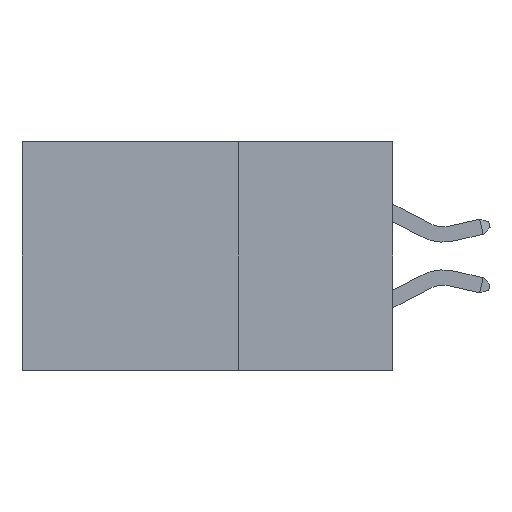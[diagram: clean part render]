
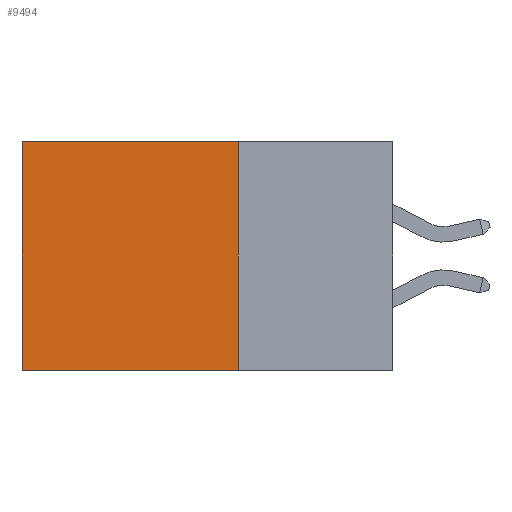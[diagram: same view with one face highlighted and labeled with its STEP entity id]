
A CAD part, left-side view. The second image highlights one B-rep face of the part: STEP entity #9494.
In plain terms, the highlighted planar face has unit normal (-1, 0, 0).
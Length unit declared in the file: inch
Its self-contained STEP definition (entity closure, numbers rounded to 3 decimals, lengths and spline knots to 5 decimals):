
#13 = CARTESIAN_POINT ( 'NONE',  ( 0.2875, 0.25, 0. ) ) ;
#37 = DIRECTION ( 'NONE',  ( 0., 0., -1. ) ) ;
#105 = ORIENTED_EDGE ( 'NONE', *, *, #1785, .T. ) ;
#1599 = EDGE_CURVE ( 'NONE', #8302, #7192, #10492, .T. ) ;
#1776 = VERTEX_POINT ( 'NONE', #13 ) ;
#1785 = EDGE_CURVE ( 'NONE', #1776, #11393, #3729, .T. ) ;
#2001 = LINE ( 'NONE', #6952, #3976 ) ;
#2182 = CARTESIAN_POINT ( 'NONE',  ( 0.2875, 0.25, -0.37 ) ) ;
#2454 = ORIENTED_EDGE ( 'NONE', *, *, #1599, .F. ) ;
#3083 = DIRECTION ( 'NONE',  ( 0., 1., 0. ) ) ;
#3729 = LINE ( 'NONE', #11576, #9092 ) ;
#3802 = DIRECTION ( 'NONE',  ( 0., 0., -1. ) ) ;
#3976 = VECTOR ( 'NONE', #7928, 39.37008 ) ;
#4517 = EDGE_CURVE ( 'NONE', #11393, #7192, #9019, .T. ) ;
#4982 = CARTESIAN_POINT ( 'NONE',  ( 0.2875, 0.25, -0.37 ) ) ;
#5694 = CARTESIAN_POINT ( 'NONE',  ( 0.2875, 0.25, 0. ) ) ;
#5913 = CARTESIAN_POINT ( 'NONE',  ( 0.2875, 0.6, 0. ) ) ;
#6952 = CARTESIAN_POINT ( 'NONE',  ( 0.2875, 0.25, 0. ) ) ;
#7192 = VERTEX_POINT ( 'NONE', #9740 ) ;
#7623 = PLANE ( 'NONE',  #8102 ) ;
#7928 = DIRECTION ( 'NONE',  ( 0., 0., -1. ) ) ;
#8092 = VECTOR ( 'NONE', #3083, 39.37008 ) ;
#8102 = AXIS2_PLACEMENT_3D ( 'NONE', #5694, #9473, #3802 ) ;
#8302 = VERTEX_POINT ( 'NONE', #4982 ) ;
#8812 = FACE_OUTER_BOUND ( 'NONE', #9238, .T. ) ;
#9019 = LINE ( 'NONE', #5913, #11101 ) ;
#9092 = VECTOR ( 'NONE', #11098, 39.37008 ) ;
#9209 = CARTESIAN_POINT ( 'NONE',  ( 0.2875, 0.6, 0. ) ) ;
#9238 = EDGE_LOOP ( 'NONE', ( #12116, #2454, #10010, #105 ) ) ;
#9473 = DIRECTION ( 'NONE',  ( 1., 0., 0. ) ) ;
#9494 = ADVANCED_FACE ( 'NONE', ( #8812 ), #7623, .F. ) ;
#9740 = CARTESIAN_POINT ( 'NONE',  ( 0.2875, 0.6, -0.37 ) ) ;
#10010 = ORIENTED_EDGE ( 'NONE', *, *, #11145, .F. ) ;
#10492 = LINE ( 'NONE', #2182, #8092 ) ;
#11098 = DIRECTION ( 'NONE',  ( 0., 1., 0. ) ) ;
#11101 = VECTOR ( 'NONE', #37, 39.37008 ) ;
#11145 = EDGE_CURVE ( 'NONE', #1776, #8302, #2001, .T. ) ;
#11393 = VERTEX_POINT ( 'NONE', #9209 ) ;
#11576 = CARTESIAN_POINT ( 'NONE',  ( 0.2875, 0.25, 0. ) ) ;
#12116 = ORIENTED_EDGE ( 'NONE', *, *, #4517, .T. ) ;
